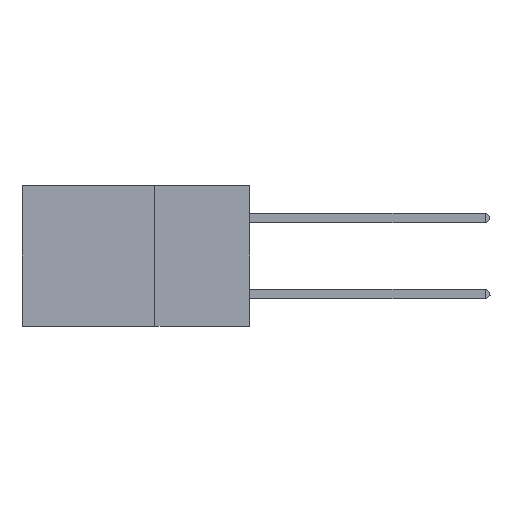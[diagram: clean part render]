
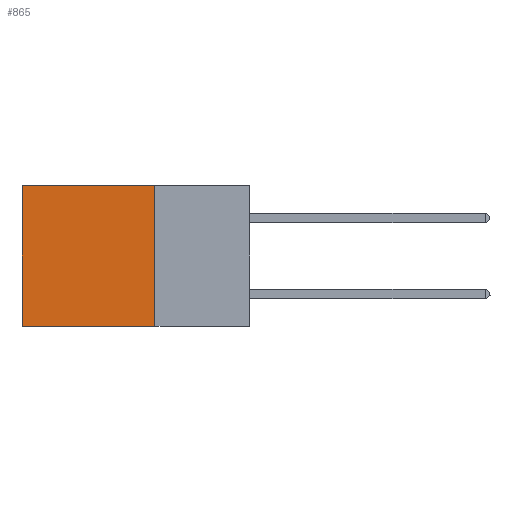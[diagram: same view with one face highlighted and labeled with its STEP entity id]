
A CAD part, left-side view. The second image highlights one B-rep face of the part: STEP entity #865.
In plain terms, the highlighted planar face has unit normal (-1, 0, 0).
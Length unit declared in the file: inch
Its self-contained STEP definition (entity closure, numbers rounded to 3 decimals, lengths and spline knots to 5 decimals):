
#44 = FACE_OUTER_BOUND ( 'NONE', #33477, .T. ) ;
#230 = PLANE ( 'NONE',  #12846 ) ;
#865 = ADVANCED_FACE ( 'NONE', ( #44 ), #230, .F. ) ;
#2425 = EDGE_CURVE ( 'NONE', #5341, #6541, #12915, .T. ) ;
#4691 = CARTESIAN_POINT ( 'NONE',  ( 0.2875, 0.6, -0.37 ) ) ;
#5341 = VERTEX_POINT ( 'NONE', #21309 ) ;
#5815 = CARTESIAN_POINT ( 'NONE',  ( 0.2875, 0.25, -0.37 ) ) ;
#6496 = VERTEX_POINT ( 'NONE', #5815 ) ;
#6541 = VERTEX_POINT ( 'NONE', #29252 ) ;
#6715 = DIRECTION ( 'NONE',  ( 0., 0., -1. ) ) ;
#10031 = DIRECTION ( 'NONE',  ( 0., 1., 0. ) ) ;
#11374 = ORIENTED_EDGE ( 'NONE', *, *, #20355, .T. ) ;
#12158 = DIRECTION ( 'NONE',  ( 1., 0., 0. ) ) ;
#12846 = AXIS2_PLACEMENT_3D ( 'NONE', #17184, #12158, #29456 ) ;
#12915 = LINE ( 'NONE', #36359, #20759 ) ;
#15336 = DIRECTION ( 'NONE',  ( 0., 0., -1. ) ) ;
#15706 = LINE ( 'NONE', #36254, #28152 ) ;
#17184 = CARTESIAN_POINT ( 'NONE',  ( 0.2875, 0.25, 0. ) ) ;
#17442 = ORIENTED_EDGE ( 'NONE', *, *, #29473, .F. ) ;
#17462 = VECTOR ( 'NONE', #6715, 39.37008 ) ;
#18340 = ORIENTED_EDGE ( 'NONE', *, *, #2425, .T. ) ;
#18356 = VERTEX_POINT ( 'NONE', #4691 ) ;
#19014 = LINE ( 'NONE', #27658, #17462 ) ;
#20355 = EDGE_CURVE ( 'NONE', #6541, #18356, #19014, .T. ) ;
#20759 = VECTOR ( 'NONE', #10031, 39.37008 ) ;
#21309 = CARTESIAN_POINT ( 'NONE',  ( 0.2875, 0.25, 0. ) ) ;
#22356 = CARTESIAN_POINT ( 'NONE',  ( 0.2875, 0.25, -0.37 ) ) ;
#27658 = CARTESIAN_POINT ( 'NONE',  ( 0.2875, 0.6, 0. ) ) ;
#28152 = VECTOR ( 'NONE', #15336, 39.37008 ) ;
#29252 = CARTESIAN_POINT ( 'NONE',  ( 0.2875, 0.6, 0. ) ) ;
#29456 = DIRECTION ( 'NONE',  ( 0., 0., -1. ) ) ;
#29473 = EDGE_CURVE ( 'NONE', #5341, #6496, #15706, .T. ) ;
#30423 = EDGE_CURVE ( 'NONE', #6496, #18356, #31184, .T. ) ;
#31184 = LINE ( 'NONE', #22356, #31909 ) ;
#31909 = VECTOR ( 'NONE', #34062, 39.37008 ) ;
#33477 = EDGE_LOOP ( 'NONE', ( #11374, #33669, #17442, #18340 ) ) ;
#33669 = ORIENTED_EDGE ( 'NONE', *, *, #30423, .F. ) ;
#34062 = DIRECTION ( 'NONE',  ( 0., 1., 0. ) ) ;
#36254 = CARTESIAN_POINT ( 'NONE',  ( 0.2875, 0.25, 0. ) ) ;
#36359 = CARTESIAN_POINT ( 'NONE',  ( 0.2875, 0.25, 0. ) ) ;
